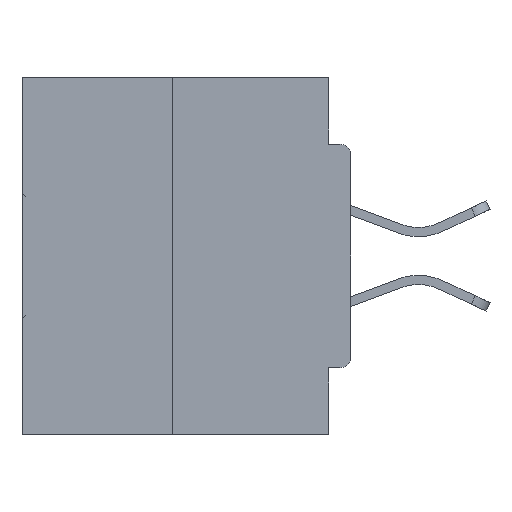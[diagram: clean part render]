
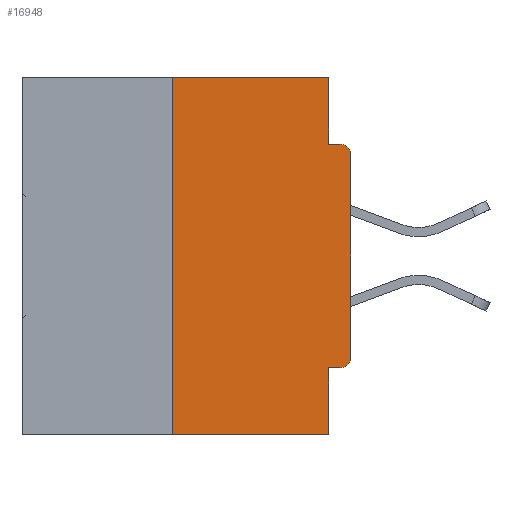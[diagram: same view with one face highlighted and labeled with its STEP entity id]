
A CAD part, left-side view. The second image highlights one B-rep face of the part: STEP entity #16948.
In plain terms, the highlighted planar face has unit normal (-1, 0, 0).
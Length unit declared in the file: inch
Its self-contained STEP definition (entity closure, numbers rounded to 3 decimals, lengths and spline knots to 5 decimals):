
#139 = ORIENTED_EDGE ( 'NONE', *, *, #18767, .F. ) ;
#1523 = VECTOR ( 'NONE', #18841, 39.37008 ) ;
#1726 = CARTESIAN_POINT ( 'NONE',  ( 0., 0.46, -0.5 ) ) ;
#2147 = LINE ( 'NONE', #12245, #9878 ) ;
#4248 = CARTESIAN_POINT ( 'NONE',  ( 0., 0.031, 0. ) ) ;
#4452 = LINE ( 'NONE', #21688, #16996 ) ;
#5131 = CARTESIAN_POINT ( 'NONE',  ( 0., 0.015, -0.1085 ) ) ;
#5708 = CARTESIAN_POINT ( 'NONE',  ( 0., 0.015, -0.3915 ) ) ;
#6279 = EDGE_CURVE ( 'NONE', #40677, #30093, #38740, .T. ) ;
#6885 = CARTESIAN_POINT ( 'NONE',  ( 0., 0.031, -0.5 ) ) ;
#7124 = CARTESIAN_POINT ( 'NONE',  ( 0., 0.46, 0. ) ) ;
#8377 = VERTEX_POINT ( 'NONE', #6885 ) ;
#8971 = DIRECTION ( 'NONE',  ( 0., 0., -1. ) ) ;
#9332 = CARTESIAN_POINT ( 'NONE',  ( 0., 0.25, 0. ) ) ;
#9878 = VECTOR ( 'NONE', #8971, 39.37008 ) ;
#10596 = CARTESIAN_POINT ( 'NONE',  ( 0., 0., -0.3915 ) ) ;
#10859 = FACE_OUTER_BOUND ( 'NONE', #21610, .T. ) ;
#10889 = EDGE_CURVE ( 'NONE', #37610, #41980, #4452, .T. ) ;
#12148 = CARTESIAN_POINT ( 'NONE',  ( 0., 0.46, 0. ) ) ;
#12245 = CARTESIAN_POINT ( 'NONE',  ( 0., 0.031, -0.5 ) ) ;
#12281 = DIRECTION ( 'NONE',  ( -1., 0., 0. ) ) ;
#12684 = VECTOR ( 'NONE', #38306, 39.37008 ) ;
#12969 = AXIS2_PLACEMENT_3D ( 'NONE', #5131, #25021, #38409 ) ;
#14139 = CIRCLE ( 'NONE', #38643, 0.015 ) ;
#14965 = CARTESIAN_POINT ( 'NONE',  ( 0., 0., -0.0935 ) ) ;
#15054 = DIRECTION ( 'NONE',  ( 0., -1., 0. ) ) ;
#15174 = VECTOR ( 'NONE', #39761, 39.37008 ) ;
#15448 = ORIENTED_EDGE ( 'NONE', *, *, #43243, .F. ) ;
#15682 = CARTESIAN_POINT ( 'NONE',  ( 0., 0., -0.1085 ) ) ;
#15837 = DIRECTION ( 'NONE',  ( 0., -1., 0. ) ) ;
#16273 = VERTEX_POINT ( 'NONE', #18196 ) ;
#16948 = ADVANCED_FACE ( 'NONE', ( #10859 ), #37347, .F. ) ;
#16996 = VECTOR ( 'NONE', #17807, 39.37008 ) ;
#17108 = EDGE_CURVE ( 'NONE', #30093, #16273, #34911, .T. ) ;
#17186 = DIRECTION ( 'NONE',  ( 1., 0., 0. ) ) ;
#17194 = ORIENTED_EDGE ( 'NONE', *, *, #22594, .T. ) ;
#17807 = DIRECTION ( 'NONE',  ( 0., 1., 0. ) ) ;
#18196 = CARTESIAN_POINT ( 'NONE',  ( 0., 0.015, -0.0935 ) ) ;
#18430 = CARTESIAN_POINT ( 'NONE',  ( 0., 0., 0. ) ) ;
#18559 = ORIENTED_EDGE ( 'NONE', *, *, #37880, .F. ) ;
#18767 = EDGE_CURVE ( 'NONE', #28360, #40677, #35567, .T. ) ;
#18841 = DIRECTION ( 'NONE',  ( 0., 0., 1. ) ) ;
#19161 = LINE ( 'NONE', #9332, #15174 ) ;
#21610 = EDGE_LOOP ( 'NONE', ( #139, #18559, #24839, #15448, #38911, #17194, #37446, #30085, #41846, #38921 ) ) ;
#21688 = CARTESIAN_POINT ( 'NONE',  ( 0., 0., -0.4065 ) ) ;
#21796 = CARTESIAN_POINT ( 'NONE',  ( 0., 0.25, 0. ) ) ;
#22594 = EDGE_CURVE ( 'NONE', #37610, #31473, #14139, .T. ) ;
#22721 = CIRCLE ( 'NONE', #12969, 0.015 ) ;
#23984 = VECTOR ( 'NONE', #38217, 39.37008 ) ;
#24839 = ORIENTED_EDGE ( 'NONE', *, *, #33126, .T. ) ;
#25021 = DIRECTION ( 'NONE',  ( -1., 0., 0. ) ) ;
#25234 = EDGE_CURVE ( 'NONE', #28459, #16273, #22721, .T. ) ;
#25390 = DIRECTION ( 'NONE',  ( 0., 0., -1. ) ) ;
#25492 = VECTOR ( 'NONE', #15837, 39.37008 ) ;
#26829 = EDGE_CURVE ( 'NONE', #31473, #28459, #29144, .T. ) ;
#27697 = VECTOR ( 'NONE', #15054, 39.37008 ) ;
#28360 = VERTEX_POINT ( 'NONE', #21796 ) ;
#28459 = VERTEX_POINT ( 'NONE', #15682 ) ;
#29144 = LINE ( 'NONE', #18430, #1523 ) ;
#30085 = ORIENTED_EDGE ( 'NONE', *, *, #25234, .T. ) ;
#30093 = VERTEX_POINT ( 'NONE', #32285 ) ;
#31473 = VERTEX_POINT ( 'NONE', #10596 ) ;
#32285 = CARTESIAN_POINT ( 'NONE',  ( 0., 0.031, -0.0935 ) ) ;
#33126 = EDGE_CURVE ( 'NONE', #38064, #8377, #38498, .T. ) ;
#34911 = LINE ( 'NONE', #14965, #23984 ) ;
#35567 = LINE ( 'NONE', #12148, #25492 ) ;
#36900 = CARTESIAN_POINT ( 'NONE',  ( 0., 0.25, -0.5 ) ) ;
#37347 = PLANE ( 'NONE',  #38037 ) ;
#37446 = ORIENTED_EDGE ( 'NONE', *, *, #26829, .T. ) ;
#37610 = VERTEX_POINT ( 'NONE', #40025 ) ;
#37767 = DIRECTION ( 'NONE',  ( 0., 0., -1. ) ) ;
#37880 = EDGE_CURVE ( 'NONE', #38064, #28360, #19161, .T. ) ;
#38037 = AXIS2_PLACEMENT_3D ( 'NONE', #7124, #17186, #37767 ) ;
#38064 = VERTEX_POINT ( 'NONE', #36900 ) ;
#38099 = CARTESIAN_POINT ( 'NONE',  ( 0., 0.031, 0. ) ) ;
#38217 = DIRECTION ( 'NONE',  ( 0., -1., 0. ) ) ;
#38306 = DIRECTION ( 'NONE',  ( 0., 0., -1. ) ) ;
#38409 = DIRECTION ( 'NONE',  ( 0., 0., -1. ) ) ;
#38498 = LINE ( 'NONE', #1726, #27697 ) ;
#38643 = AXIS2_PLACEMENT_3D ( 'NONE', #5708, #12281, #25390 ) ;
#38740 = LINE ( 'NONE', #38099, #12684 ) ;
#38858 = CARTESIAN_POINT ( 'NONE',  ( 0., 0.031, -0.4065 ) ) ;
#38911 = ORIENTED_EDGE ( 'NONE', *, *, #10889, .F. ) ;
#38921 = ORIENTED_EDGE ( 'NONE', *, *, #6279, .F. ) ;
#39761 = DIRECTION ( 'NONE',  ( 0., 0., 1. ) ) ;
#40025 = CARTESIAN_POINT ( 'NONE',  ( 0., 0.015, -0.4065 ) ) ;
#40677 = VERTEX_POINT ( 'NONE', #4248 ) ;
#41846 = ORIENTED_EDGE ( 'NONE', *, *, #17108, .F. ) ;
#41980 = VERTEX_POINT ( 'NONE', #38858 ) ;
#43243 = EDGE_CURVE ( 'NONE', #41980, #8377, #2147, .T. ) ;
